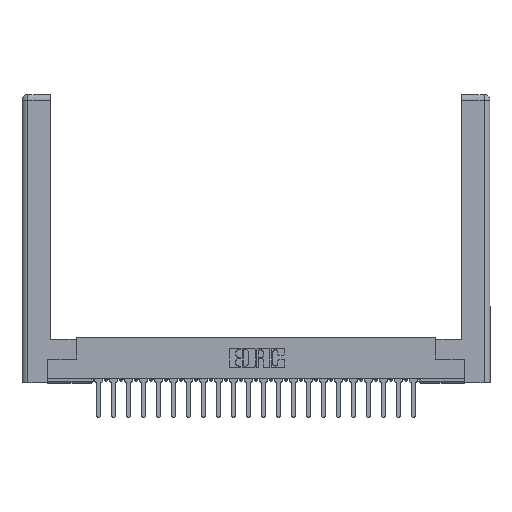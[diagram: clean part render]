
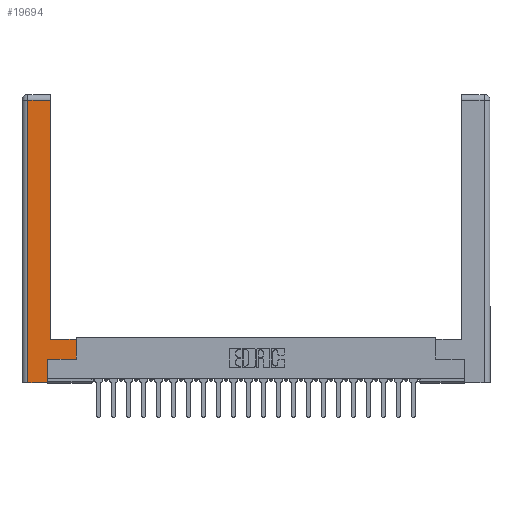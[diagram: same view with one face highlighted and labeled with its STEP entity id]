
A CAD part, top view. The second image highlights one B-rep face of the part: STEP entity #19694.
In plain terms, the highlighted planar face has unit normal (0, 0, 1).
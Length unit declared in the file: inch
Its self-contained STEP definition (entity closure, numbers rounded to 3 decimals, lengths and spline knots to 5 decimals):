
#151 = DIRECTION ( 'NONE',  ( 0., 0., -1. ) ) ;
#394 = FACE_OUTER_BOUND ( 'NONE', #9069, .T. ) ;
#622 = VERTEX_POINT ( 'NONE', #20029 ) ;
#750 = LINE ( 'NONE', #4673, #10487 ) ;
#1019 = CARTESIAN_POINT ( 'NONE',  ( 0.565, 0.245, 0. ) ) ;
#1565 = EDGE_CURVE ( 'NONE', #15444, #622, #7841, .T. ) ;
#1572 = DIRECTION ( 'NONE',  ( 1., 0., 0. ) ) ;
#2482 = DIRECTION ( 'NONE',  ( 0., -1., 0. ) ) ;
#3687 = DIRECTION ( 'NONE',  ( 0., 1., 0. ) ) ;
#4045 = LINE ( 'NONE', #20247, #22402 ) ;
#4057 = ORIENTED_EDGE ( 'NONE', *, *, #12318, .T. ) ;
#4211 = DIRECTION ( 'NONE',  ( 0., 1., 0. ) ) ;
#4673 = CARTESIAN_POINT ( 'NONE',  ( 0.265, 0.245, 0. ) ) ;
#5036 = CARTESIAN_POINT ( 'NONE',  ( 0.265, 0., 0. ) ) ;
#5061 = EDGE_CURVE ( 'NONE', #20520, #22456, #21204, .T. ) ;
#5223 = VECTOR ( 'NONE', #15569, 39.37008 ) ;
#5229 = LINE ( 'NONE', #18176, #19772 ) ;
#5298 = VECTOR ( 'NONE', #4211, 39.37008 ) ;
#5876 = PLANE ( 'NONE',  #20224 ) ;
#7102 = EDGE_CURVE ( 'NONE', #14983, #15444, #5229, .T. ) ;
#7827 = ORIENTED_EDGE ( 'NONE', *, *, #5061, .T. ) ;
#7841 = LINE ( 'NONE', #18961, #5298 ) ;
#8230 = CARTESIAN_POINT ( 'NONE',  ( 0.295, 0.45, 0. ) ) ;
#9069 = EDGE_LOOP ( 'NONE', ( #21091, #7827, #17119, #4057, #23559, #9829, #10625, #18302 ) ) ;
#9211 = CARTESIAN_POINT ( 'NONE',  ( 0.0615, 2.94, 0. ) ) ;
#9829 = ORIENTED_EDGE ( 'NONE', *, *, #7102, .T. ) ;
#9849 = VERTEX_POINT ( 'NONE', #22987 ) ;
#9921 = VECTOR ( 'NONE', #10484, 39.37008 ) ;
#10312 = EDGE_CURVE ( 'NONE', #622, #9849, #11600, .T. ) ;
#10451 = DIRECTION ( 'NONE',  ( -1., 0., 0. ) ) ;
#10484 = DIRECTION ( 'NONE',  ( 1., 0., 0. ) ) ;
#10487 = VECTOR ( 'NONE', #12154, 39.37008 ) ;
#10625 = ORIENTED_EDGE ( 'NONE', *, *, #1565, .T. ) ;
#11600 = LINE ( 'NONE', #8230, #5223 ) ;
#12154 = DIRECTION ( 'NONE',  ( 0., 1., 0. ) ) ;
#12318 = EDGE_CURVE ( 'NONE', #17675, #19533, #23290, .T. ) ;
#12671 = LINE ( 'NONE', #16529, #23635 ) ;
#14983 = VERTEX_POINT ( 'NONE', #17307 ) ;
#15444 = VERTEX_POINT ( 'NONE', #1019 ) ;
#15569 = DIRECTION ( 'NONE',  ( -1., 0., 0. ) ) ;
#16529 = CARTESIAN_POINT ( 'NONE',  ( 0.0615, 0., 0. ) ) ;
#17119 = ORIENTED_EDGE ( 'NONE', *, *, #18725, .T. ) ;
#17307 = CARTESIAN_POINT ( 'NONE',  ( 0.265, 0.245, 0. ) ) ;
#17418 = EDGE_CURVE ( 'NONE', #9849, #20520, #4045, .T. ) ;
#17675 = VERTEX_POINT ( 'NONE', #19759 ) ;
#17696 = CARTESIAN_POINT ( 'NONE',  ( 0.0615, 2.94, 0. ) ) ;
#18176 = CARTESIAN_POINT ( 'NONE',  ( 0.565, 0.245, 0. ) ) ;
#18302 = ORIENTED_EDGE ( 'NONE', *, *, #10312, .T. ) ;
#18725 = EDGE_CURVE ( 'NONE', #22456, #17675, #12671, .T. ) ;
#18961 = CARTESIAN_POINT ( 'NONE',  ( 0.565, 0.45, 0. ) ) ;
#19497 = VECTOR ( 'NONE', #10451, 39.37008 ) ;
#19533 = VERTEX_POINT ( 'NONE', #20034 ) ;
#19694 = ADVANCED_FACE ( 'NONE', ( #394 ), #5876, .F. ) ;
#19759 = CARTESIAN_POINT ( 'NONE',  ( 0.0615, 0., 0. ) ) ;
#19772 = VECTOR ( 'NONE', #1572, 39.37008 ) ;
#20029 = CARTESIAN_POINT ( 'NONE',  ( 0.565, 0.45, 0. ) ) ;
#20034 = CARTESIAN_POINT ( 'NONE',  ( 0.265, 0., 0. ) ) ;
#20224 = AXIS2_PLACEMENT_3D ( 'NONE', #22554, #151, #22440 ) ;
#20247 = CARTESIAN_POINT ( 'NONE',  ( 0.295, 3., 0. ) ) ;
#20520 = VERTEX_POINT ( 'NONE', #21312 ) ;
#21091 = ORIENTED_EDGE ( 'NONE', *, *, #17418, .T. ) ;
#21204 = LINE ( 'NONE', #17696, #19497 ) ;
#21305 = EDGE_CURVE ( 'NONE', #19533, #14983, #750, .T. ) ;
#21312 = CARTESIAN_POINT ( 'NONE',  ( 0.295, 2.94, 0. ) ) ;
#22402 = VECTOR ( 'NONE', #3687, 39.37008 ) ;
#22440 = DIRECTION ( 'NONE',  ( -1., 0., 0. ) ) ;
#22456 = VERTEX_POINT ( 'NONE', #9211 ) ;
#22554 = CARTESIAN_POINT ( 'NONE',  ( 0., 0., 0. ) ) ;
#22987 = CARTESIAN_POINT ( 'NONE',  ( 0.295, 0.45, 0. ) ) ;
#23290 = LINE ( 'NONE', #5036, #9921 ) ;
#23559 = ORIENTED_EDGE ( 'NONE', *, *, #21305, .T. ) ;
#23635 = VECTOR ( 'NONE', #2482, 39.37008 ) ;
